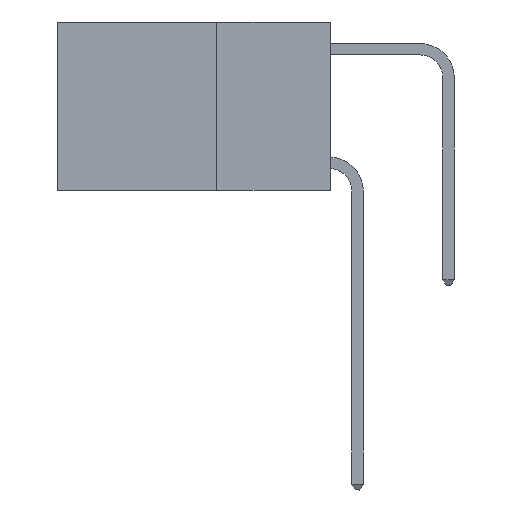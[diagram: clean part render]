
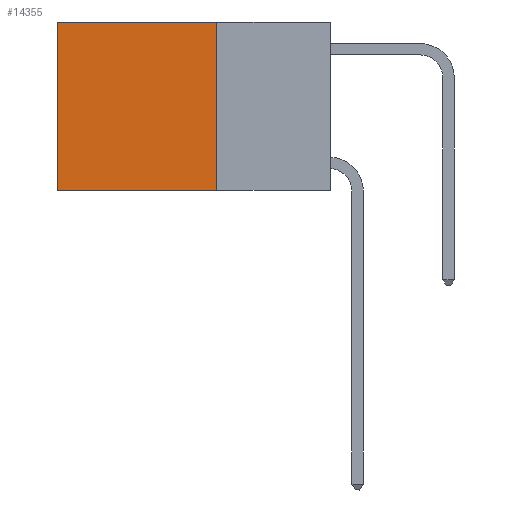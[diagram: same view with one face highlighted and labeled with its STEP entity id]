
A CAD part, left-side view. The second image highlights one B-rep face of the part: STEP entity #14355.
In plain terms, the highlighted planar face has unit normal (-1, 0, 0).
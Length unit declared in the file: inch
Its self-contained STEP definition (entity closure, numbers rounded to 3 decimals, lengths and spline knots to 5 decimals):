
#1198 = CARTESIAN_POINT ( 'NONE',  ( 0.2625, 0.25, 0. ) ) ;
#1329 = VERTEX_POINT ( 'NONE', #4055 ) ;
#1782 = VERTEX_POINT ( 'NONE', #12955 ) ;
#1975 = CARTESIAN_POINT ( 'NONE',  ( 0.2625, 0.25, 0. ) ) ;
#3169 = EDGE_CURVE ( 'NONE', #13560, #1329, #4023, .T. ) ;
#3448 = DIRECTION ( 'NONE',  ( 0., 0., -1. ) ) ;
#3676 = VECTOR ( 'NONE', #11074, 39.37008 ) ;
#3982 = CARTESIAN_POINT ( 'NONE',  ( 0.2625, 0.25, 0. ) ) ;
#3998 = CARTESIAN_POINT ( 'NONE',  ( 0.2625, 0.25, 0. ) ) ;
#4023 = LINE ( 'NONE', #9939, #3676 ) ;
#4055 = CARTESIAN_POINT ( 'NONE',  ( 0.2625, 0.6, -0.37 ) ) ;
#4109 = VECTOR ( 'NONE', #9545, 39.37008 ) ;
#5527 = LINE ( 'NONE', #3982, #14113 ) ;
#5566 = EDGE_LOOP ( 'NONE', ( #12502, #11274, #11279, #9893 ) ) ;
#6114 = EDGE_CURVE ( 'NONE', #13596, #1782, #5527, .T. ) ;
#6771 = CARTESIAN_POINT ( 'NONE',  ( 0.2625, 0.6, 0. ) ) ;
#7235 = DIRECTION ( 'NONE',  ( 0., 1., 0. ) ) ;
#7462 = CARTESIAN_POINT ( 'NONE',  ( 0.2625, 0.25, -0.37 ) ) ;
#7795 = LINE ( 'NONE', #6771, #13783 ) ;
#7887 = PLANE ( 'NONE',  #9362 ) ;
#9362 = AXIS2_PLACEMENT_3D ( 'NONE', #1198, #10124, #3448 ) ;
#9545 = DIRECTION ( 'NONE',  ( 0., 0., -1. ) ) ;
#9893 = ORIENTED_EDGE ( 'NONE', *, *, #6114, .T. ) ;
#9939 = CARTESIAN_POINT ( 'NONE',  ( 0.2625, 0.25, -0.37 ) ) ;
#10124 = DIRECTION ( 'NONE',  ( 1., 0., 0. ) ) ;
#10454 = EDGE_CURVE ( 'NONE', #1782, #1329, #7795, .T. ) ;
#11074 = DIRECTION ( 'NONE',  ( 0., 1., 0. ) ) ;
#11274 = ORIENTED_EDGE ( 'NONE', *, *, #3169, .F. ) ;
#11279 = ORIENTED_EDGE ( 'NONE', *, *, #12083, .F. ) ;
#12083 = EDGE_CURVE ( 'NONE', #13596, #13560, #13040, .T. ) ;
#12406 = DIRECTION ( 'NONE',  ( 0., 0., -1. ) ) ;
#12502 = ORIENTED_EDGE ( 'NONE', *, *, #10454, .T. ) ;
#12955 = CARTESIAN_POINT ( 'NONE',  ( 0.2625, 0.6, 0. ) ) ;
#13040 = LINE ( 'NONE', #3998, #4109 ) ;
#13053 = FACE_OUTER_BOUND ( 'NONE', #5566, .T. ) ;
#13560 = VERTEX_POINT ( 'NONE', #7462 ) ;
#13596 = VERTEX_POINT ( 'NONE', #1975 ) ;
#13783 = VECTOR ( 'NONE', #12406, 39.37008 ) ;
#14113 = VECTOR ( 'NONE', #7235, 39.37008 ) ;
#14355 = ADVANCED_FACE ( 'NONE', ( #13053 ), #7887, .F. ) ;
